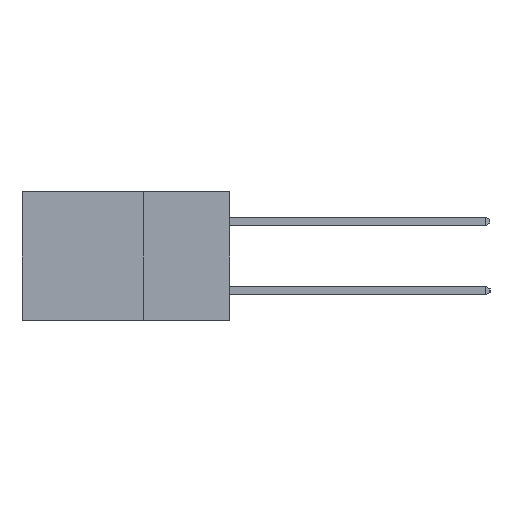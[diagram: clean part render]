
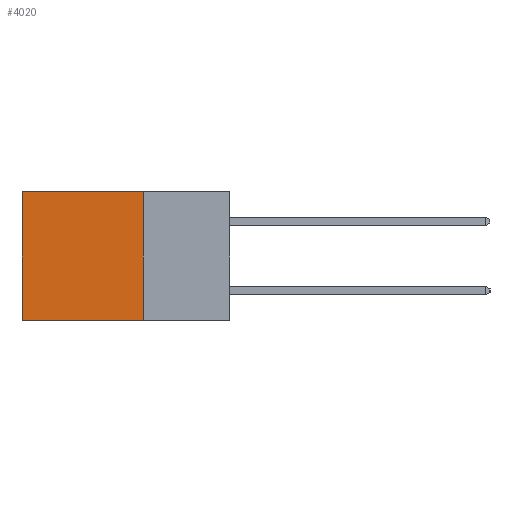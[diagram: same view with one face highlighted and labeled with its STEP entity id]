
A CAD part, left-side view. The second image highlights one B-rep face of the part: STEP entity #4020.
In plain terms, the highlighted planar face has unit normal (-1, 0, 0).
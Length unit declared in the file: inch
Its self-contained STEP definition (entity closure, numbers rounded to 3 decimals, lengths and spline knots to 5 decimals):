
#467 = DIRECTION ( 'NONE',  ( 0., 0., -1. ) ) ;
#654 = CARTESIAN_POINT ( 'NONE',  ( 0.2615, 0.6, -0.37 ) ) ;
#1008 = EDGE_CURVE ( 'NONE', #3598, #12936, #7572, .T. ) ;
#1157 = DIRECTION ( 'NONE',  ( 0., 1., 0. ) ) ;
#1445 = EDGE_CURVE ( 'NONE', #8565, #10828, #5432, .T. ) ;
#1636 = EDGE_CURVE ( 'NONE', #12936, #10828, #6411, .T. ) ;
#2090 = CARTESIAN_POINT ( 'NONE',  ( 0.2615, 0.25, 0. ) ) ;
#2120 = CARTESIAN_POINT ( 'NONE',  ( 0.2615, 0.6, 0. ) ) ;
#2315 = EDGE_LOOP ( 'NONE', ( #3125, #6382, #6532, #8240 ) ) ;
#2545 = CARTESIAN_POINT ( 'NONE',  ( 0.2615, 0.25, 0. ) ) ;
#2875 = EDGE_CURVE ( 'NONE', #3598, #8565, #12626, .T. ) ;
#3123 = AXIS2_PLACEMENT_3D ( 'NONE', #6425, #6412, #6379 ) ;
#3125 = ORIENTED_EDGE ( 'NONE', *, *, #1636, .T. ) ;
#3571 = VECTOR ( 'NONE', #467, 39.37008 ) ;
#3598 = VERTEX_POINT ( 'NONE', #2545 ) ;
#3675 = CARTESIAN_POINT ( 'NONE',  ( 0.2615, 0.25, -0.37 ) ) ;
#3722 = CARTESIAN_POINT ( 'NONE',  ( 0.2615, 0.6, -0.37 ) ) ;
#3866 = DIRECTION ( 'NONE',  ( 0., 1., 0. ) ) ;
#3952 = DIRECTION ( 'NONE',  ( 0., 0., -1. ) ) ;
#4020 = ADVANCED_FACE ( 'NONE', ( #11647 ), #7422, .F. ) ;
#5432 = LINE ( 'NONE', #6065, #12805 ) ;
#6065 = CARTESIAN_POINT ( 'NONE',  ( 0.2615, 0.25, -0.37 ) ) ;
#6379 = DIRECTION ( 'NONE',  ( 0., 0., -1. ) ) ;
#6382 = ORIENTED_EDGE ( 'NONE', *, *, #1445, .F. ) ;
#6411 = LINE ( 'NONE', #654, #3571 ) ;
#6412 = DIRECTION ( 'NONE',  ( 1., 0., 0. ) ) ;
#6425 = CARTESIAN_POINT ( 'NONE',  ( 0.2615, 0.25, -0.37 ) ) ;
#6532 = ORIENTED_EDGE ( 'NONE', *, *, #2875, .F. ) ;
#7422 = PLANE ( 'NONE',  #3123 ) ;
#7572 = LINE ( 'NONE', #2090, #10461 ) ;
#8240 = ORIENTED_EDGE ( 'NONE', *, *, #1008, .T. ) ;
#8565 = VERTEX_POINT ( 'NONE', #8788 ) ;
#8788 = CARTESIAN_POINT ( 'NONE',  ( 0.2615, 0.25, -0.37 ) ) ;
#10243 = VECTOR ( 'NONE', #3952, 39.37008 ) ;
#10461 = VECTOR ( 'NONE', #1157, 39.37008 ) ;
#10828 = VERTEX_POINT ( 'NONE', #3722 ) ;
#11647 = FACE_OUTER_BOUND ( 'NONE', #2315, .T. ) ;
#12626 = LINE ( 'NONE', #3675, #10243 ) ;
#12805 = VECTOR ( 'NONE', #3866, 39.37008 ) ;
#12936 = VERTEX_POINT ( 'NONE', #2120 ) ;
